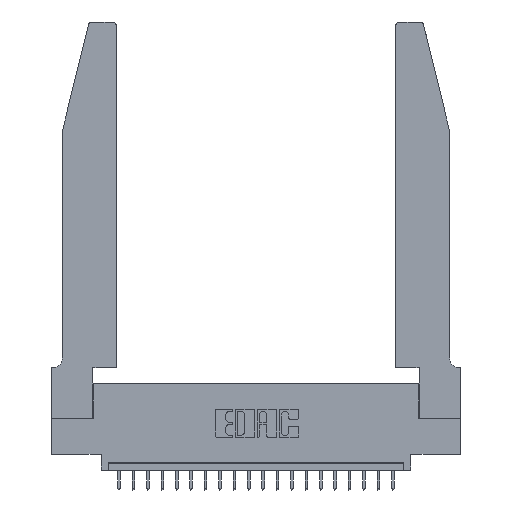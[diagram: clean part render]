
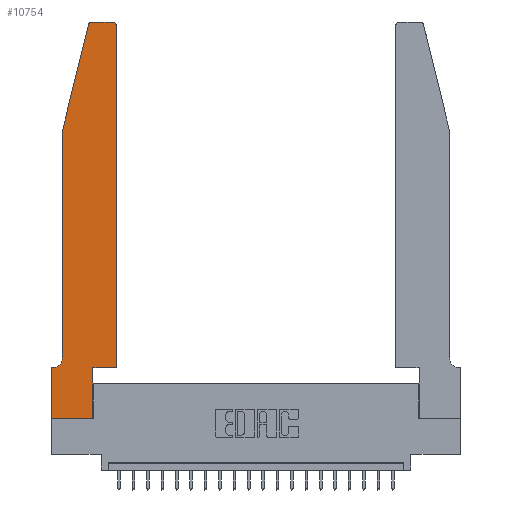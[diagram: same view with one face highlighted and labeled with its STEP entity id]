
A CAD part, top view. The second image highlights one B-rep face of the part: STEP entity #10754.
In plain terms, the highlighted planar face has unit normal (0, 0, 1).
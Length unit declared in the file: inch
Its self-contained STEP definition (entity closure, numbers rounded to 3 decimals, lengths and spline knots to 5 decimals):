
#165 = ORIENTED_EDGE ( 'NONE', *, *, #20673, .T. ) ;
#421 = CARTESIAN_POINT ( 'NONE',  ( 0., 0., 0.37 ) ) ;
#731 = DIRECTION ( 'NONE',  ( 1., 0., 0. ) ) ;
#874 = LINE ( 'NONE', #6317, #2101 ) ;
#1138 = VERTEX_POINT ( 'NONE', #18283 ) ;
#1374 = DIRECTION ( 'NONE',  ( 1., 0., 0. ) ) ;
#1893 = DIRECTION ( 'NONE',  ( 1., 0., 0. ) ) ;
#1918 = VERTEX_POINT ( 'NONE', #2501 ) ;
#2099 = VECTOR ( 'NONE', #5839, 39.37008 ) ;
#2101 = VECTOR ( 'NONE', #11598, 39.37008 ) ;
#2181 = ORIENTED_EDGE ( 'NONE', *, *, #18882, .T. ) ;
#2501 = CARTESIAN_POINT ( 'NONE',  ( 0.25487, 2.72718, 0.37 ) ) ;
#2640 = CARTESIAN_POINT ( 'NONE',  ( 0.4505, 0.35, 0.37 ) ) ;
#2834 = VERTEX_POINT ( 'NONE', #8212 ) ;
#3041 = ORIENTED_EDGE ( 'NONE', *, *, #16033, .T. ) ;
#3318 = CARTESIAN_POINT ( 'NONE',  ( 0.284, 2.75, 0.37 ) ) ;
#3393 = EDGE_LOOP ( 'NONE', ( #12590, #3041, #8846, #2181, #10973, #165, #9538, #9546, #6844, #21437, #12985, #15220 ) ) ;
#3425 = VERTEX_POINT ( 'NONE', #11716 ) ;
#3683 = CARTESIAN_POINT ( 'NONE',  ( 0.0055, 0.42, 0.37 ) ) ;
#3793 = CARTESIAN_POINT ( 'NONE',  ( 0., 0.35, 0.37 ) ) ;
#4171 = VERTEX_POINT ( 'NONE', #18310 ) ;
#4535 = CIRCLE ( 'NONE', #18692, 0.03 ) ;
#5552 = DIRECTION ( 'NONE',  ( -0.239, -0.971, 0. ) ) ;
#5823 = DIRECTION ( 'NONE',  ( 0., 0., 1. ) ) ;
#5839 = DIRECTION ( 'NONE',  ( 0., -1., 0. ) ) ;
#6317 = CARTESIAN_POINT ( 'NONE',  ( 0.4505, 0.35, 0.37 ) ) ;
#6367 = LINE ( 'NONE', #22648, #17614 ) ;
#6550 = VECTOR ( 'NONE', #14705, 39.37008 ) ;
#6844 = ORIENTED_EDGE ( 'NONE', *, *, #16762, .T. ) ;
#7247 = CARTESIAN_POINT ( 'NONE',  ( 0., 0., 0.37 ) ) ;
#8033 = CARTESIAN_POINT ( 'NONE',  ( 0.0055, 0.35, 0.37 ) ) ;
#8212 = CARTESIAN_POINT ( 'NONE',  ( 0.2865, 0., 0.37 ) ) ;
#8372 = CARTESIAN_POINT ( 'NONE',  ( 0., 0.35, 0.37 ) ) ;
#8382 = VERTEX_POINT ( 'NONE', #10919 ) ;
#8539 = VERTEX_POINT ( 'NONE', #15882 ) ;
#8674 = DIRECTION ( 'NONE',  ( 0., 0., 1. ) ) ;
#8703 = CARTESIAN_POINT ( 'NONE',  ( 0.0755, 2., 0.37 ) ) ;
#8846 = ORIENTED_EDGE ( 'NONE', *, *, #17182, .T. ) ;
#9032 = LINE ( 'NONE', #421, #22668 ) ;
#9166 = AXIS2_PLACEMENT_3D ( 'NONE', #3683, #18342, #21926 ) ;
#9538 = ORIENTED_EDGE ( 'NONE', *, *, #22036, .T. ) ;
#9546 = ORIENTED_EDGE ( 'NONE', *, *, #11141, .T. ) ;
#9675 = VERTEX_POINT ( 'NONE', #8033 ) ;
#9876 = LINE ( 'NONE', #2640, #6550 ) ;
#9884 = VECTOR ( 'NONE', #14108, 39.37008 ) ;
#9960 = LINE ( 'NONE', #17726, #18091 ) ;
#10116 = PLANE ( 'NONE',  #16030 ) ;
#10368 = VERTEX_POINT ( 'NONE', #3793 ) ;
#10442 = LINE ( 'NONE', #8703, #9884 ) ;
#10754 = ADVANCED_FACE ( 'NONE', ( #21888 ), #10116, .T. ) ;
#10919 = CARTESIAN_POINT ( 'NONE',  ( 0.4505, 0.35, 0.37 ) ) ;
#10973 = ORIENTED_EDGE ( 'NONE', *, *, #21304, .T. ) ;
#11019 = CIRCLE ( 'NONE', #9166, 0.07 ) ;
#11141 = EDGE_CURVE ( 'NONE', #22630, #2834, #9032, .T. ) ;
#11598 = DIRECTION ( 'NONE',  ( 1., 0., 0. ) ) ;
#11716 = CARTESIAN_POINT ( 'NONE',  ( 0.0755, 2., 0.37 ) ) ;
#12412 = AXIS2_PLACEMENT_3D ( 'NONE', #18966, #13801, #1374 ) ;
#12590 = ORIENTED_EDGE ( 'NONE', *, *, #17264, .T. ) ;
#12707 = LINE ( 'NONE', #16069, #22422 ) ;
#12985 = ORIENTED_EDGE ( 'NONE', *, *, #21891, .T. ) ;
#13204 = CIRCLE ( 'NONE', #12412, 0.03 ) ;
#13590 = LINE ( 'NONE', #17157, #17244 ) ;
#13801 = DIRECTION ( 'NONE',  ( 0., 0., 1. ) ) ;
#14108 = DIRECTION ( 'NONE',  ( 0., -1., 0. ) ) ;
#14644 = LINE ( 'NONE', #7247, #2099 ) ;
#14705 = DIRECTION ( 'NONE',  ( 0., 1., 0. ) ) ;
#14918 = CARTESIAN_POINT ( 'NONE',  ( 0.4205, 2.75, 0.37 ) ) ;
#15220 = ORIENTED_EDGE ( 'NONE', *, *, #17424, .T. ) ;
#15652 = CARTESIAN_POINT ( 'NONE',  ( 0.284, 2.72, 0.37 ) ) ;
#15882 = CARTESIAN_POINT ( 'NONE',  ( 0.0755, 0.42, 0.37 ) ) ;
#15883 = DIRECTION ( 'NONE',  ( -1., 0., 0. ) ) ;
#16030 = AXIS2_PLACEMENT_3D ( 'NONE', #8372, #5823, #731 ) ;
#16033 = EDGE_CURVE ( 'NONE', #18878, #1918, #4535, .T. ) ;
#16069 = CARTESIAN_POINT ( 'NONE',  ( 0.0755, 2., 0.37 ) ) ;
#16144 = DIRECTION ( 'NONE',  ( 1., 0., 0. ) ) ;
#16228 = CARTESIAN_POINT ( 'NONE',  ( 0., 0., 0.37 ) ) ;
#16762 = EDGE_CURVE ( 'NONE', #2834, #4171, #13590, .T. ) ;
#17157 = CARTESIAN_POINT ( 'NONE',  ( 0.2865, 0.35, 0.37 ) ) ;
#17182 = EDGE_CURVE ( 'NONE', #1918, #3425, #12707, .T. ) ;
#17244 = VECTOR ( 'NONE', #20592, 39.37008 ) ;
#17264 = EDGE_CURVE ( 'NONE', #22887, #18878, #6367, .T. ) ;
#17424 = EDGE_CURVE ( 'NONE', #1138, #22887, #13204, .T. ) ;
#17614 = VECTOR ( 'NONE', #20884, 39.37008 ) ;
#17726 = CARTESIAN_POINT ( 'NONE',  ( 0.0755, 0.35, 0.37 ) ) ;
#18091 = VECTOR ( 'NONE', #15883, 39.37008 ) ;
#18283 = CARTESIAN_POINT ( 'NONE',  ( 0.4505, 2.72, 0.37 ) ) ;
#18310 = CARTESIAN_POINT ( 'NONE',  ( 0.2865, 0.35, 0.37 ) ) ;
#18342 = DIRECTION ( 'NONE',  ( 0., 0., -1. ) ) ;
#18692 = AXIS2_PLACEMENT_3D ( 'NONE', #15652, #8674, #1893 ) ;
#18878 = VERTEX_POINT ( 'NONE', #3318 ) ;
#18882 = EDGE_CURVE ( 'NONE', #3425, #8539, #10442, .T. ) ;
#18966 = CARTESIAN_POINT ( 'NONE',  ( 0.4205, 2.72, 0.37 ) ) ;
#20592 = DIRECTION ( 'NONE',  ( 0., 1., 0. ) ) ;
#20644 = EDGE_CURVE ( 'NONE', #4171, #8382, #874, .T. ) ;
#20673 = EDGE_CURVE ( 'NONE', #9675, #10368, #9960, .T. ) ;
#20884 = DIRECTION ( 'NONE',  ( -1., 0., 0. ) ) ;
#21304 = EDGE_CURVE ( 'NONE', #8539, #9675, #11019, .T. ) ;
#21437 = ORIENTED_EDGE ( 'NONE', *, *, #20644, .T. ) ;
#21888 = FACE_OUTER_BOUND ( 'NONE', #3393, .T. ) ;
#21891 = EDGE_CURVE ( 'NONE', #8382, #1138, #9876, .T. ) ;
#21926 = DIRECTION ( 'NONE',  ( -1., 0., 0. ) ) ;
#22036 = EDGE_CURVE ( 'NONE', #10368, #22630, #14644, .T. ) ;
#22422 = VECTOR ( 'NONE', #5552, 39.37008 ) ;
#22630 = VERTEX_POINT ( 'NONE', #16228 ) ;
#22648 = CARTESIAN_POINT ( 'NONE',  ( 0.2605, 2.75, 0.37 ) ) ;
#22668 = VECTOR ( 'NONE', #16144, 39.37008 ) ;
#22887 = VERTEX_POINT ( 'NONE', #14918 ) ;
